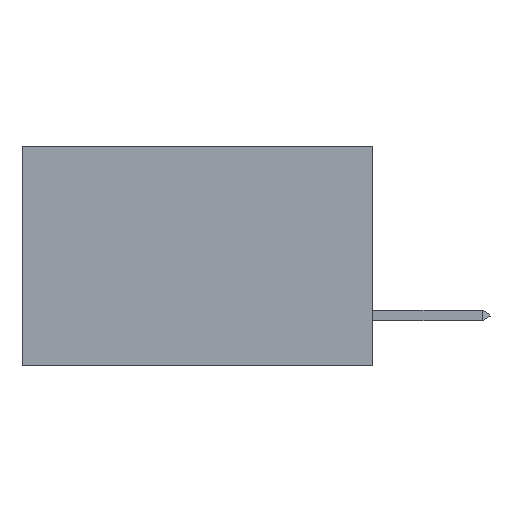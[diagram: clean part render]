
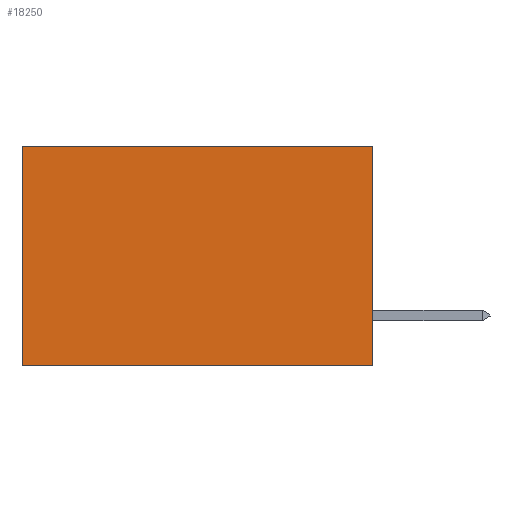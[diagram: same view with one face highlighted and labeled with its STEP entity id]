
A CAD part, left-side view. The second image highlights one B-rep face of the part: STEP entity #18250.
In plain terms, the highlighted planar face has unit normal (-1, 0, 0).
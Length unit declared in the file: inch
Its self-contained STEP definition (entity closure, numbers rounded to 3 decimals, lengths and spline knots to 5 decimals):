
#1114 = VERTEX_POINT ( 'NONE', #13047 ) ;
#1629 = CARTESIAN_POINT ( 'NONE',  ( 0.277, 0., -0.37 ) ) ;
#1903 = VERTEX_POINT ( 'NONE', #15183 ) ;
#2592 = CARTESIAN_POINT ( 'NONE',  ( 0.277, 0., 0. ) ) ;
#3207 = DIRECTION ( 'NONE',  ( 1., 0., 0. ) ) ;
#4835 = EDGE_CURVE ( 'NONE', #1114, #10816, #9273, .T. ) ;
#5086 = EDGE_CURVE ( 'NONE', #5833, #1114, #18477, .T. ) ;
#5434 = VECTOR ( 'NONE', #15366, 39.37008 ) ;
#5479 = LINE ( 'NONE', #17346, #16368 ) ;
#5489 = DIRECTION ( 'NONE',  ( 0., 1., 0. ) ) ;
#5833 = VERTEX_POINT ( 'NONE', #2592 ) ;
#6776 = AXIS2_PLACEMENT_3D ( 'NONE', #1629, #3207, #13271 ) ;
#7426 = DIRECTION ( 'NONE',  ( 0., 0., -1. ) ) ;
#7760 = EDGE_CURVE ( 'NONE', #1903, #10816, #9095, .T. ) ;
#8011 = EDGE_CURVE ( 'NONE', #5833, #1903, #5479, .T. ) ;
#8432 = ORIENTED_EDGE ( 'NONE', *, *, #4835, .T. ) ;
#9095 = LINE ( 'NONE', #14067, #9562 ) ;
#9273 = LINE ( 'NONE', #15423, #5434 ) ;
#9562 = VECTOR ( 'NONE', #5489, 39.37008 ) ;
#10412 = PLANE ( 'NONE',  #6776 ) ;
#10816 = VERTEX_POINT ( 'NONE', #12796 ) ;
#11676 = DIRECTION ( 'NONE',  ( 0., 1., 0. ) ) ;
#11800 = CARTESIAN_POINT ( 'NONE',  ( 0.277, 0., 0. ) ) ;
#12796 = CARTESIAN_POINT ( 'NONE',  ( 0.277, 0.59, -0.37 ) ) ;
#13047 = CARTESIAN_POINT ( 'NONE',  ( 0.277, 0.59, 0. ) ) ;
#13271 = DIRECTION ( 'NONE',  ( 0., 0., -1. ) ) ;
#14067 = CARTESIAN_POINT ( 'NONE',  ( 0.277, 0., -0.37 ) ) ;
#14179 = ORIENTED_EDGE ( 'NONE', *, *, #7760, .F. ) ;
#14312 = ORIENTED_EDGE ( 'NONE', *, *, #8011, .F. ) ;
#14787 = VECTOR ( 'NONE', #11676, 39.37008 ) ;
#15183 = CARTESIAN_POINT ( 'NONE',  ( 0.277, 0., -0.37 ) ) ;
#15366 = DIRECTION ( 'NONE',  ( 0., 0., -1. ) ) ;
#15423 = CARTESIAN_POINT ( 'NONE',  ( 0.277, 0.59, -0.37 ) ) ;
#16368 = VECTOR ( 'NONE', #7426, 39.37008 ) ;
#16768 = FACE_OUTER_BOUND ( 'NONE', #16982, .T. ) ;
#16982 = EDGE_LOOP ( 'NONE', ( #8432, #14179, #14312, #17557 ) ) ;
#17346 = CARTESIAN_POINT ( 'NONE',  ( 0.277, 0., -0.37 ) ) ;
#17557 = ORIENTED_EDGE ( 'NONE', *, *, #5086, .T. ) ;
#18250 = ADVANCED_FACE ( 'NONE', ( #16768 ), #10412, .F. ) ;
#18477 = LINE ( 'NONE', #11800, #14787 ) ;
